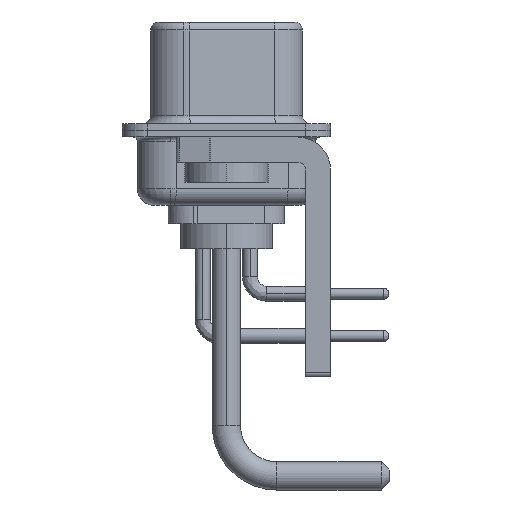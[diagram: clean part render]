
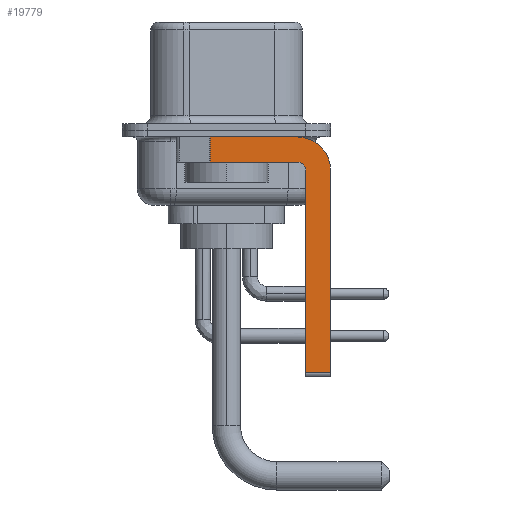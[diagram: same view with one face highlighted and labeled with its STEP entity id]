
A CAD part, left-side view. The second image highlights one B-rep face of the part: STEP entity #19779.
In plain terms, the highlighted planar face has unit normal (-1, 0, 0).
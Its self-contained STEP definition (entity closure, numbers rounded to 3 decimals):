
#1002 = VECTOR ( 'NONE', #1544, 1000. ) ;
#1544 = DIRECTION ( 'NONE',  ( 0., 0., -1. ) ) ;
#1634 = VERTEX_POINT ( 'NONE', #13907 ) ;
#1692 = VECTOR ( 'NONE', #14294, 1000. ) ;
#2093 = PLANE ( 'NONE',  #7518 ) ;
#2447 = CARTESIAN_POINT ( 'NONE',  ( -2.9, -4.25, -2.4 ) ) ;
#2843 = ORIENTED_EDGE ( 'NONE', *, *, #6062, .F. ) ;
#3148 = DIRECTION ( 'NONE',  ( -1., 0., 0. ) ) ;
#3688 = LINE ( 'NONE', #12309, #1002 ) ;
#5755 = ORIENTED_EDGE ( 'NONE', *, *, #11827, .F. ) ;
#5878 = DIRECTION ( 'NONE',  ( 0., 0., -1. ) ) ;
#6062 = EDGE_CURVE ( 'NONE', #1634, #8542, #17763, .T. ) ;
#6537 = ORIENTED_EDGE ( 'NONE', *, *, #14247, .F. ) ;
#7214 = EDGE_LOOP ( 'NONE', ( #22803, #19363, #18314, #2843, #22114, #13140, #6537, #5755 ) ) ;
#7274 = CARTESIAN_POINT ( 'NONE',  ( -2.9, -4.25, -2.4 ) ) ;
#7518 = AXIS2_PLACEMENT_3D ( 'NONE', #2447, #7669, #5878 ) ;
#7669 = DIRECTION ( 'NONE',  ( 1., 0., 0. ) ) ;
#7747 = VERTEX_POINT ( 'NONE', #18308 ) ;
#7752 = DIRECTION ( 'NONE',  ( 0., 0., -1. ) ) ;
#8455 = CARTESIAN_POINT ( 'NONE',  ( -2.9, -4.75, -14.8 ) ) ;
#8542 = VERTEX_POINT ( 'NONE', #12799 ) ;
#10354 = DIRECTION ( 'NONE',  ( 0., 0., 1. ) ) ;
#10412 = EDGE_CURVE ( 'NONE', #23222, #22642, #3688, .T. ) ;
#10435 = CARTESIAN_POINT ( 'NONE',  ( -2.9, -4.75, -14.55 ) ) ;
#10911 = DIRECTION ( 'NONE',  ( 0., -1., 0. ) ) ;
#11159 = VECTOR ( 'NONE', #20444, 1000. ) ;
#11514 = EDGE_CURVE ( 'NONE', #15026, #7747, #12212, .T. ) ;
#11629 = AXIS2_PLACEMENT_3D ( 'NONE', #14728, #21710, #7752 ) ;
#11633 = VECTOR ( 'NONE', #15661, 1000. ) ;
#11827 = EDGE_CURVE ( 'NONE', #14946, #20800, #15008, .T. ) ;
#11867 = LINE ( 'NONE', #8455, #11633 ) ;
#12212 = LINE ( 'NONE', #15905, #13709 ) ;
#12309 = CARTESIAN_POINT ( 'NONE',  ( -2.9, 0.978, -1.9 ) ) ;
#12392 = CARTESIAN_POINT ( 'NONE',  ( -2.9, -4.25, -1.9 ) ) ;
#12799 = CARTESIAN_POINT ( 'NONE',  ( -2.9, -4.25, -1.9 ) ) ;
#13044 = VECTOR ( 'NONE', #19621, 1000. ) ;
#13140 = ORIENTED_EDGE ( 'NONE', *, *, #11514, .T. ) ;
#13332 = CARTESIAN_POINT ( 'NONE',  ( -2.9, 3., -0.4 ) ) ;
#13709 = VECTOR ( 'NONE', #10911, 1000. ) ;
#13907 = CARTESIAN_POINT ( 'NONE',  ( -2.9, -4.75, -2.4 ) ) ;
#14096 = CARTESIAN_POINT ( 'NONE',  ( -2.9, -4.25, -0.4 ) ) ;
#14156 = CARTESIAN_POINT ( 'NONE',  ( -2.9, 0.978, -0.4 ) ) ;
#14247 = EDGE_CURVE ( 'NONE', #20800, #7747, #17853, .T. ) ;
#14267 = CARTESIAN_POINT ( 'NONE',  ( -2.9, 0.978, -1.9 ) ) ;
#14294 = DIRECTION ( 'NONE',  ( 0., 0., -1. ) ) ;
#14728 = CARTESIAN_POINT ( 'NONE',  ( -2.9, -4.25, -2.4 ) ) ;
#14759 = FACE_OUTER_BOUND ( 'NONE', #7214, .T. ) ;
#14946 = VERTEX_POINT ( 'NONE', #14096 ) ;
#15008 = CIRCLE ( 'NONE', #11629, 2. ) ;
#15026 = VERTEX_POINT ( 'NONE', #10435 ) ;
#15661 = DIRECTION ( 'NONE',  ( 0., 0., 1. ) ) ;
#15905 = CARTESIAN_POINT ( 'NONE',  ( -2.9, -4.25, -14.55 ) ) ;
#16131 = EDGE_CURVE ( 'NONE', #8542, #22642, #21388, .T. ) ;
#16482 = EDGE_CURVE ( 'NONE', #23222, #14946, #22213, .T. ) ;
#17763 = CIRCLE ( 'NONE', #18545, 0.5 ) ;
#17853 = LINE ( 'NONE', #23296, #1692 ) ;
#18308 = CARTESIAN_POINT ( 'NONE',  ( -2.9, -6.25, -14.55 ) ) ;
#18314 = ORIENTED_EDGE ( 'NONE', *, *, #16131, .F. ) ;
#18545 = AXIS2_PLACEMENT_3D ( 'NONE', #7274, #3148, #10354 ) ;
#19363 = ORIENTED_EDGE ( 'NONE', *, *, #10412, .T. ) ;
#19621 = DIRECTION ( 'NONE',  ( 0., 1., 0. ) ) ;
#19779 = ADVANCED_FACE ( 'NONE', ( #14759 ), #2093, .F. ) ;
#20444 = DIRECTION ( 'NONE',  ( 0., -1., 0. ) ) ;
#20500 = EDGE_CURVE ( 'NONE', #15026, #1634, #11867, .T. ) ;
#20800 = VERTEX_POINT ( 'NONE', #22041 ) ;
#21388 = LINE ( 'NONE', #12392, #13044 ) ;
#21710 = DIRECTION ( 'NONE',  ( 1., 0., 0. ) ) ;
#22041 = CARTESIAN_POINT ( 'NONE',  ( -2.9, -6.25, -2.4 ) ) ;
#22114 = ORIENTED_EDGE ( 'NONE', *, *, #20500, .F. ) ;
#22213 = LINE ( 'NONE', #13332, #11159 ) ;
#22642 = VERTEX_POINT ( 'NONE', #14267 ) ;
#22803 = ORIENTED_EDGE ( 'NONE', *, *, #16482, .F. ) ;
#23222 = VERTEX_POINT ( 'NONE', #14156 ) ;
#23296 = CARTESIAN_POINT ( 'NONE',  ( -2.9, -6.25, -2.4 ) ) ;
